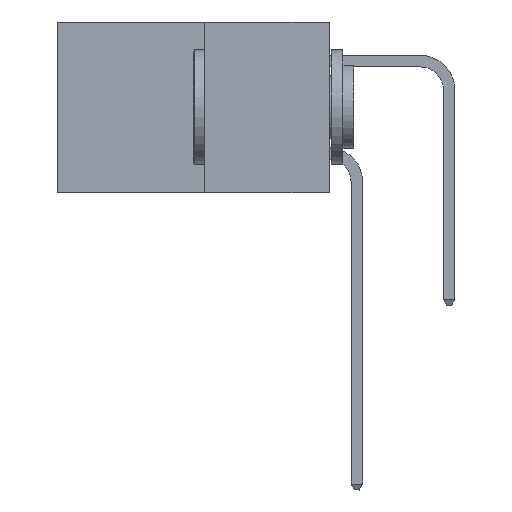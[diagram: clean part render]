
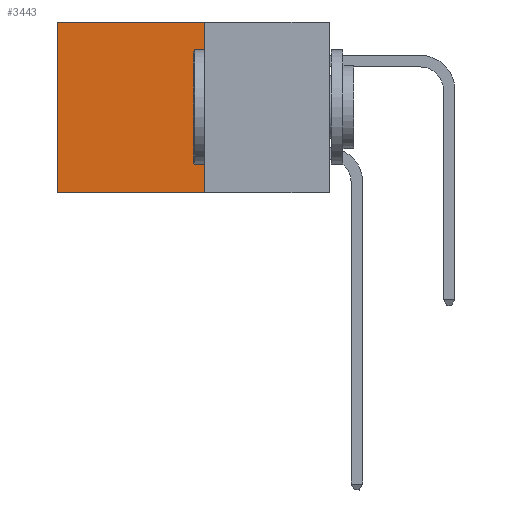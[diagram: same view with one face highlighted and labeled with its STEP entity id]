
A CAD part, left-side view. The second image highlights one B-rep face of the part: STEP entity #3443.
In plain terms, the highlighted planar face has unit normal (-1, 0, 0).
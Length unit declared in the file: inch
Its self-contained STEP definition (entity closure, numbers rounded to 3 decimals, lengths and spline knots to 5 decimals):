
#479 = DIRECTION ( 'NONE',  ( 0., 0., -1. ) ) ;
#2402 = ORIENTED_EDGE ( 'NONE', *, *, #19023, .T. ) ;
#3443 = ADVANCED_FACE ( 'NONE', ( #18694 ), #12070, .F. ) ;
#4314 = VECTOR ( 'NONE', #18629, 39.37008 ) ;
#4598 = VERTEX_POINT ( 'NONE', #31898 ) ;
#6380 = AXIS2_PLACEMENT_3D ( 'NONE', #10472, #9303, #30571 ) ;
#6887 = EDGE_CURVE ( 'NONE', #4598, #15489, #28047, .T. ) ;
#7522 = LINE ( 'NONE', #15839, #30984 ) ;
#9303 = DIRECTION ( 'NONE',  ( 1., 0., 0. ) ) ;
#10472 = CARTESIAN_POINT ( 'NONE',  ( 0.277, 0.27, -0.37 ) ) ;
#11213 = VERTEX_POINT ( 'NONE', #18038 ) ;
#12070 = PLANE ( 'NONE',  #6380 ) ;
#14805 = CARTESIAN_POINT ( 'NONE',  ( 0.277, 0.27, -0.37 ) ) ;
#15334 = CARTESIAN_POINT ( 'NONE',  ( 0.277, 0.59, -0.37 ) ) ;
#15489 = VERTEX_POINT ( 'NONE', #15334 ) ;
#15839 = CARTESIAN_POINT ( 'NONE',  ( 0.277, 0.27, -0.37 ) ) ;
#17237 = CARTESIAN_POINT ( 'NONE',  ( 0.277, 0.59, -0.37 ) ) ;
#18038 = CARTESIAN_POINT ( 'NONE',  ( 0.277, 0.27, 0. ) ) ;
#18629 = DIRECTION ( 'NONE',  ( 0., 1., 0. ) ) ;
#18694 = FACE_OUTER_BOUND ( 'NONE', #30803, .T. ) ;
#18959 = EDGE_CURVE ( 'NONE', #11213, #4598, #7522, .T. ) ;
#19023 = EDGE_CURVE ( 'NONE', #11213, #30763, #31418, .T. ) ;
#21625 = ORIENTED_EDGE ( 'NONE', *, *, #6887, .F. ) ;
#25363 = VECTOR ( 'NONE', #30038, 39.37008 ) ;
#27266 = VECTOR ( 'NONE', #32521, 39.37008 ) ;
#27635 = ORIENTED_EDGE ( 'NONE', *, *, #27803, .T. ) ;
#27636 = CARTESIAN_POINT ( 'NONE',  ( 0.277, 0.59, 0. ) ) ;
#27803 = EDGE_CURVE ( 'NONE', #30763, #15489, #32047, .T. ) ;
#28047 = LINE ( 'NONE', #14805, #27266 ) ;
#28232 = ORIENTED_EDGE ( 'NONE', *, *, #18959, .F. ) ;
#30038 = DIRECTION ( 'NONE',  ( 0., 0., -1. ) ) ;
#30571 = DIRECTION ( 'NONE',  ( 0., 0., -1. ) ) ;
#30763 = VERTEX_POINT ( 'NONE', #27636 ) ;
#30803 = EDGE_LOOP ( 'NONE', ( #27635, #21625, #28232, #2402 ) ) ;
#30984 = VECTOR ( 'NONE', #479, 39.37008 ) ;
#31256 = CARTESIAN_POINT ( 'NONE',  ( 0.277, 0.27, 0. ) ) ;
#31418 = LINE ( 'NONE', #31256, #4314 ) ;
#31898 = CARTESIAN_POINT ( 'NONE',  ( 0.277, 0.27, -0.37 ) ) ;
#32047 = LINE ( 'NONE', #17237, #25363 ) ;
#32521 = DIRECTION ( 'NONE',  ( 0., 1., 0. ) ) ;
